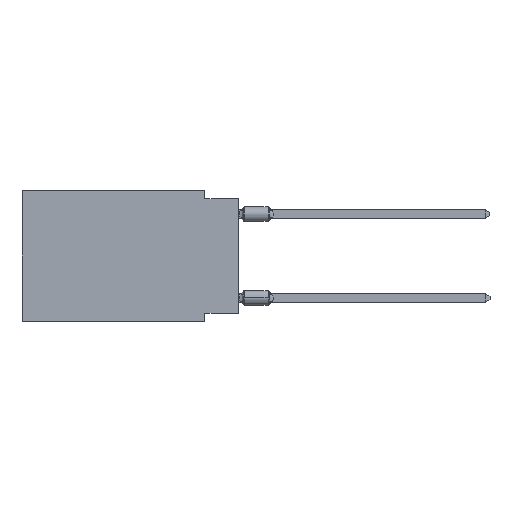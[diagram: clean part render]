
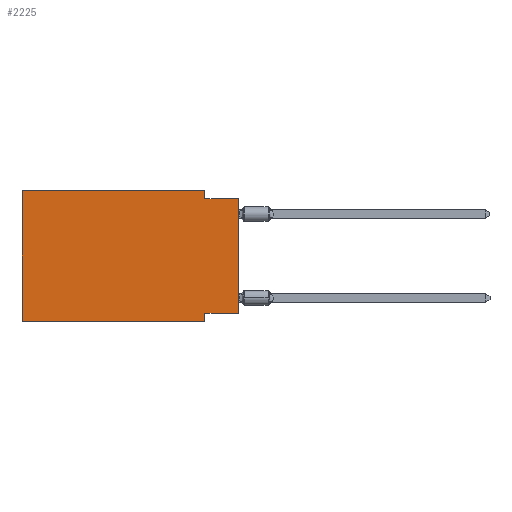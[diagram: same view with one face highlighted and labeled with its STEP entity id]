
A CAD part, left-side view. The second image highlights one B-rep face of the part: STEP entity #2225.
In plain terms, the highlighted planar face has unit normal (-1, 0, 0).
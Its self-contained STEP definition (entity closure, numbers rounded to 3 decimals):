
#253 = CARTESIAN_POINT ( 'NONE',  ( 0., 2.54, -9.271 ) ) ;
#556 = CARTESIAN_POINT ( 'NONE',  ( 0., 0., -9.271 ) ) ;
#588 = VERTEX_POINT ( 'NONE', #11382 ) ;
#665 = DIRECTION ( 'NONE',  ( 0., 0., -1. ) ) ;
#858 = VECTOR ( 'NONE', #9458, 1000. ) ;
#1751 = EDGE_LOOP ( 'NONE', ( #7413, #2247, #7952, #14065, #7243, #13287, #14019, #13590 ) ) ;
#2003 = DIRECTION ( 'NONE',  ( 0., 0., 1. ) ) ;
#2225 = ADVANCED_FACE ( 'NONE', ( #11605 ), #12764, .F. ) ;
#2247 = ORIENTED_EDGE ( 'NONE', *, *, #6632, .F. ) ;
#2886 = EDGE_CURVE ( 'NONE', #4934, #3794, #11072, .T. ) ;
#2904 = LINE ( 'NONE', #8555, #12578 ) ;
#2947 = LINE ( 'NONE', #7435, #5639 ) ;
#3202 = AXIS2_PLACEMENT_3D ( 'NONE', #8481, #3916, #7180 ) ;
#3794 = VERTEX_POINT ( 'NONE', #7167 ) ;
#3806 = CARTESIAN_POINT ( 'NONE',  ( 0., 2.54, 0. ) ) ;
#3916 = DIRECTION ( 'NONE',  ( 1., 0., 0. ) ) ;
#4259 = CARTESIAN_POINT ( 'NONE',  ( 0., 2.54, -9.906 ) ) ;
#4262 = DIRECTION ( 'NONE',  ( 0., 0., 1. ) ) ;
#4459 = VECTOR ( 'NONE', #665, 1000. ) ;
#4934 = VERTEX_POINT ( 'NONE', #10024 ) ;
#4991 = DIRECTION ( 'NONE',  ( 0., -1., 0. ) ) ;
#5164 = DIRECTION ( 'NONE',  ( 0., -1., 0. ) ) ;
#5211 = LINE ( 'NONE', #9910, #10927 ) ;
#5639 = VECTOR ( 'NONE', #6288, 1000. ) ;
#6029 = EDGE_CURVE ( 'NONE', #6961, #4934, #10432, .T. ) ;
#6046 = EDGE_CURVE ( 'NONE', #8820, #11601, #5211, .T. ) ;
#6086 = CARTESIAN_POINT ( 'NONE',  ( 0., 16.383, 0. ) ) ;
#6288 = DIRECTION ( 'NONE',  ( 0., 1., 0. ) ) ;
#6632 = EDGE_CURVE ( 'NONE', #588, #11601, #2904, .T. ) ;
#6961 = VERTEX_POINT ( 'NONE', #13643 ) ;
#6969 = CARTESIAN_POINT ( 'NONE',  ( 0., 16.383, -9.906 ) ) ;
#7167 = CARTESIAN_POINT ( 'NONE',  ( 0., 2.54, 0. ) ) ;
#7180 = DIRECTION ( 'NONE',  ( 0., 0., -1. ) ) ;
#7243 = ORIENTED_EDGE ( 'NONE', *, *, #6029, .F. ) ;
#7413 = ORIENTED_EDGE ( 'NONE', *, *, #6046, .T. ) ;
#7435 = CARTESIAN_POINT ( 'NONE',  ( 0., 0., -9.271 ) ) ;
#7455 = VECTOR ( 'NONE', #2003, 1000. ) ;
#7952 = ORIENTED_EDGE ( 'NONE', *, *, #9251, .F. ) ;
#8353 = LINE ( 'NONE', #10604, #4459 ) ;
#8481 = CARTESIAN_POINT ( 'NONE',  ( 0., 16.383, 0. ) ) ;
#8555 = CARTESIAN_POINT ( 'NONE',  ( 0., 0., -0.635 ) ) ;
#8820 = VERTEX_POINT ( 'NONE', #556 ) ;
#9251 = EDGE_CURVE ( 'NONE', #3794, #588, #12869, .T. ) ;
#9458 = DIRECTION ( 'NONE',  ( 0., 0., -1. ) ) ;
#9910 = CARTESIAN_POINT ( 'NONE',  ( 0., 0., 0. ) ) ;
#10024 = CARTESIAN_POINT ( 'NONE',  ( 0., 16.383, 0. ) ) ;
#10040 = CARTESIAN_POINT ( 'NONE',  ( 0., 0., -0.635 ) ) ;
#10059 = DIRECTION ( 'NONE',  ( 0., -1., 0. ) ) ;
#10160 = VERTEX_POINT ( 'NONE', #253 ) ;
#10170 = VECTOR ( 'NONE', #10059, 1000. ) ;
#10198 = CARTESIAN_POINT ( 'NONE',  ( 0., 16.383, 0. ) ) ;
#10432 = LINE ( 'NONE', #6086, #7455 ) ;
#10604 = CARTESIAN_POINT ( 'NONE',  ( 0., 2.54, -9.906 ) ) ;
#10678 = EDGE_CURVE ( 'NONE', #10160, #12838, #8353, .T. ) ;
#10927 = VECTOR ( 'NONE', #4262, 1000. ) ;
#10972 = EDGE_CURVE ( 'NONE', #6961, #12838, #11187, .T. ) ;
#11047 = EDGE_CURVE ( 'NONE', #8820, #10160, #2947, .T. ) ;
#11072 = LINE ( 'NONE', #10198, #10170 ) ;
#11187 = LINE ( 'NONE', #6969, #11650 ) ;
#11382 = CARTESIAN_POINT ( 'NONE',  ( 0., 2.54, -0.635 ) ) ;
#11601 = VERTEX_POINT ( 'NONE', #10040 ) ;
#11605 = FACE_OUTER_BOUND ( 'NONE', #1751, .T. ) ;
#11650 = VECTOR ( 'NONE', #4991, 1000. ) ;
#12578 = VECTOR ( 'NONE', #5164, 1000. ) ;
#12764 = PLANE ( 'NONE',  #3202 ) ;
#12838 = VERTEX_POINT ( 'NONE', #4259 ) ;
#12869 = LINE ( 'NONE', #3806, #858 ) ;
#13287 = ORIENTED_EDGE ( 'NONE', *, *, #10972, .T. ) ;
#13590 = ORIENTED_EDGE ( 'NONE', *, *, #11047, .F. ) ;
#13643 = CARTESIAN_POINT ( 'NONE',  ( 0., 16.383, -9.906 ) ) ;
#14019 = ORIENTED_EDGE ( 'NONE', *, *, #10678, .F. ) ;
#14065 = ORIENTED_EDGE ( 'NONE', *, *, #2886, .F. ) ;
